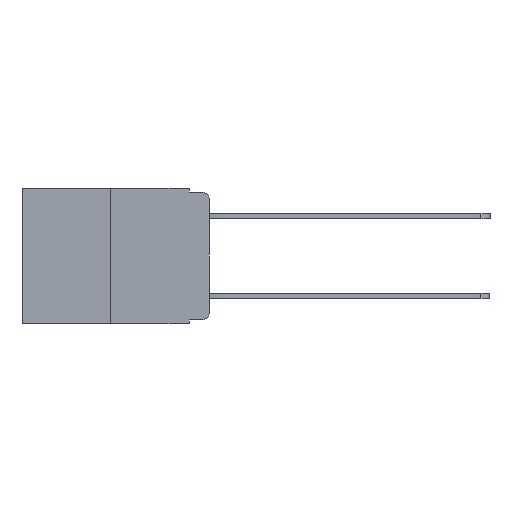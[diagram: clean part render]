
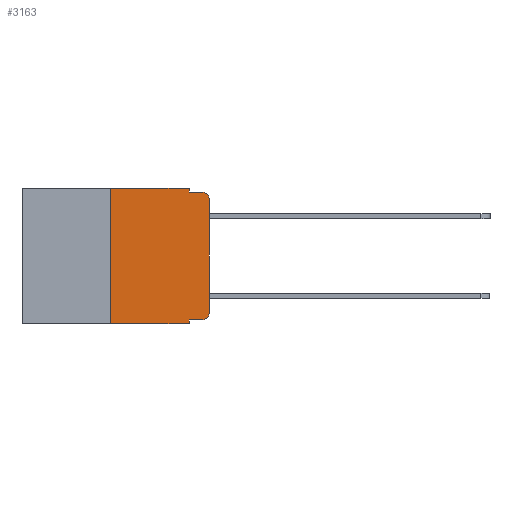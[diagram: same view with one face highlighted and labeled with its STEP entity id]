
A CAD part, left-side view. The second image highlights one B-rep face of the part: STEP entity #3163.
In plain terms, the highlighted planar face has unit normal (-1, 0, 0).
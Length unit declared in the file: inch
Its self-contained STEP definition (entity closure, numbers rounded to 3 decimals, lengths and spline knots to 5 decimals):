
#355 = VERTEX_POINT ( 'NONE', #5323 ) ;
#449 = LINE ( 'NONE', #11885, #14265 ) ;
#571 = CARTESIAN_POINT ( 'NONE',  ( 0., 0.25, 0. ) ) ;
#691 = VECTOR ( 'NONE', #16022, 39.37008 ) ;
#939 = EDGE_CURVE ( 'NONE', #2992, #11663, #5043, .T. ) ;
#999 = CARTESIAN_POINT ( 'NONE',  ( 0., 0.02, -0.313 ) ) ;
#1164 = LINE ( 'NONE', #12215, #5058 ) ;
#1419 = CARTESIAN_POINT ( 'NONE',  ( 0., 0.051, -0.333 ) ) ;
#1588 = VERTEX_POINT ( 'NONE', #12882 ) ;
#1763 = VECTOR ( 'NONE', #9347, 39.37008 ) ;
#1918 = EDGE_CURVE ( 'NONE', #2992, #14258, #449, .T. ) ;
#2222 = AXIS2_PLACEMENT_3D ( 'NONE', #999, #10782, #2462 ) ;
#2462 = DIRECTION ( 'NONE',  ( 0., 0., -1. ) ) ;
#2600 = CARTESIAN_POINT ( 'NONE',  ( 0., 0., -0.03 ) ) ;
#2702 = DIRECTION ( 'NONE',  ( 0., -1., 0. ) ) ;
#2882 = EDGE_CURVE ( 'NONE', #14230, #14176, #6103, .T. ) ;
#2975 = LINE ( 'NONE', #15445, #10019 ) ;
#2992 = VERTEX_POINT ( 'NONE', #3931 ) ;
#3163 = ADVANCED_FACE ( 'NONE', ( #12590 ), #11702, .F. ) ;
#3931 = CARTESIAN_POINT ( 'NONE',  ( 0., 0.051, -0.333 ) ) ;
#3945 = CARTESIAN_POINT ( 'NONE',  ( 0., 0.051, -0.01 ) ) ;
#4093 = CARTESIAN_POINT ( 'NONE',  ( 0., 0.25, 0. ) ) ;
#4867 = CARTESIAN_POINT ( 'NONE',  ( 0., 0.473, 0. ) ) ;
#5043 = LINE ( 'NONE', #1419, #14833 ) ;
#5058 = VECTOR ( 'NONE', #2702, 39.37008 ) ;
#5175 = ORIENTED_EDGE ( 'NONE', *, *, #939, .T. ) ;
#5323 = CARTESIAN_POINT ( 'NONE',  ( 0., 0.02, -0.01 ) ) ;
#5824 = EDGE_CURVE ( 'NONE', #12394, #15245, #13833, .T. ) ;
#5957 = DIRECTION ( 'NONE',  ( 0., 0., -1. ) ) ;
#6103 = LINE ( 'NONE', #571, #1763 ) ;
#6435 = VECTOR ( 'NONE', #13860, 39.37008 ) ;
#6711 = DIRECTION ( 'NONE',  ( 0., -1., 0. ) ) ;
#7297 = LINE ( 'NONE', #4867, #6435 ) ;
#7409 = CARTESIAN_POINT ( 'NONE',  ( 0., 0., 0. ) ) ;
#7564 = DIRECTION ( 'NONE',  ( -1., 0., 0. ) ) ;
#7628 = ORIENTED_EDGE ( 'NONE', *, *, #1918, .F. ) ;
#7688 = EDGE_CURVE ( 'NONE', #15245, #355, #1164, .T. ) ;
#7711 = AXIS2_PLACEMENT_3D ( 'NONE', #14974, #7564, #16152 ) ;
#7962 = EDGE_CURVE ( 'NONE', #14230, #14258, #2975, .T. ) ;
#8614 = EDGE_CURVE ( 'NONE', #1588, #15379, #14456, .T. ) ;
#9018 = CARTESIAN_POINT ( 'NONE',  ( 0., 0.051, 0. ) ) ;
#9093 = DIRECTION ( 'NONE',  ( 0., 0., -1. ) ) ;
#9347 = DIRECTION ( 'NONE',  ( 0., 0., 1. ) ) ;
#9520 = EDGE_CURVE ( 'NONE', #15379, #355, #15349, .T. ) ;
#9949 = ORIENTED_EDGE ( 'NONE', *, *, #5824, .F. ) ;
#10019 = VECTOR ( 'NONE', #6711, 39.37008 ) ;
#10026 = DIRECTION ( 'NONE',  ( 0., -1., 0. ) ) ;
#10373 = ORIENTED_EDGE ( 'NONE', *, *, #7962, .T. ) ;
#10465 = CARTESIAN_POINT ( 'NONE',  ( 0., 0.051, 0. ) ) ;
#10681 = VECTOR ( 'NONE', #11692, 39.37008 ) ;
#10782 = DIRECTION ( 'NONE',  ( -1., 0., 0. ) ) ;
#10896 = ORIENTED_EDGE ( 'NONE', *, *, #8614, .T. ) ;
#11049 = EDGE_LOOP ( 'NONE', ( #10896, #14208, #13866, #9949, #16619, #15330, #10373, #7628, #5175, #13895 ) ) ;
#11663 = VERTEX_POINT ( 'NONE', #14370 ) ;
#11692 = DIRECTION ( 'NONE',  ( 0., 0., -1. ) ) ;
#11702 = PLANE ( 'NONE',  #11800 ) ;
#11800 = AXIS2_PLACEMENT_3D ( 'NONE', #15926, #11946, #5957 ) ;
#11885 = CARTESIAN_POINT ( 'NONE',  ( 0., 0.051, 0. ) ) ;
#11946 = DIRECTION ( 'NONE',  ( 1., 0., 0. ) ) ;
#12215 = CARTESIAN_POINT ( 'NONE',  ( 0., 0.051, -0.01 ) ) ;
#12394 = VERTEX_POINT ( 'NONE', #9018 ) ;
#12440 = EDGE_CURVE ( 'NONE', #14176, #12394, #7297, .T. ) ;
#12590 = FACE_OUTER_BOUND ( 'NONE', #11049, .T. ) ;
#12882 = CARTESIAN_POINT ( 'NONE',  ( 0., 0., -0.313 ) ) ;
#13387 = CARTESIAN_POINT ( 'NONE',  ( 0., 0.25, -0.343 ) ) ;
#13833 = LINE ( 'NONE', #10465, #10681 ) ;
#13860 = DIRECTION ( 'NONE',  ( 0., -1., 0. ) ) ;
#13866 = ORIENTED_EDGE ( 'NONE', *, *, #7688, .F. ) ;
#13895 = ORIENTED_EDGE ( 'NONE', *, *, #16199, .T. ) ;
#14176 = VERTEX_POINT ( 'NONE', #4093 ) ;
#14208 = ORIENTED_EDGE ( 'NONE', *, *, #9520, .T. ) ;
#14230 = VERTEX_POINT ( 'NONE', #13387 ) ;
#14258 = VERTEX_POINT ( 'NONE', #16921 ) ;
#14265 = VECTOR ( 'NONE', #9093, 39.37008 ) ;
#14370 = CARTESIAN_POINT ( 'NONE',  ( 0., 0.02, -0.333 ) ) ;
#14456 = LINE ( 'NONE', #7409, #691 ) ;
#14833 = VECTOR ( 'NONE', #10026, 39.37008 ) ;
#14974 = CARTESIAN_POINT ( 'NONE',  ( 0., 0.02, -0.03 ) ) ;
#15245 = VERTEX_POINT ( 'NONE', #3945 ) ;
#15330 = ORIENTED_EDGE ( 'NONE', *, *, #2882, .F. ) ;
#15349 = CIRCLE ( 'NONE', #7711, 0.02 ) ;
#15379 = VERTEX_POINT ( 'NONE', #2600 ) ;
#15445 = CARTESIAN_POINT ( 'NONE',  ( 0., 0.473, -0.343 ) ) ;
#15557 = CIRCLE ( 'NONE', #2222, 0.02 ) ;
#15926 = CARTESIAN_POINT ( 'NONE',  ( 0., 0.473, 0. ) ) ;
#16022 = DIRECTION ( 'NONE',  ( 0., 0., 1. ) ) ;
#16152 = DIRECTION ( 'NONE',  ( 0., 0., -1. ) ) ;
#16199 = EDGE_CURVE ( 'NONE', #11663, #1588, #15557, .T. ) ;
#16619 = ORIENTED_EDGE ( 'NONE', *, *, #12440, .F. ) ;
#16921 = CARTESIAN_POINT ( 'NONE',  ( 0., 0.051, -0.343 ) ) ;
